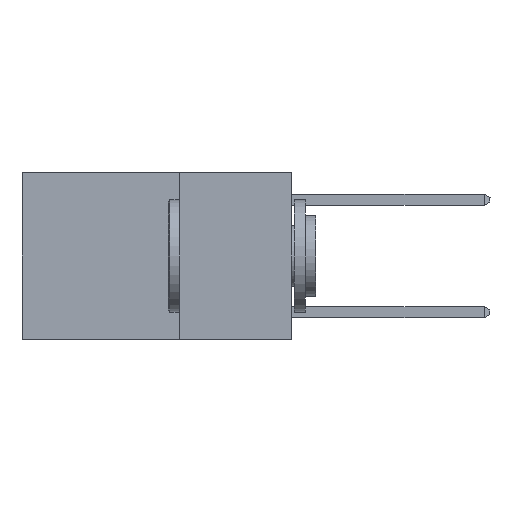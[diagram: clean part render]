
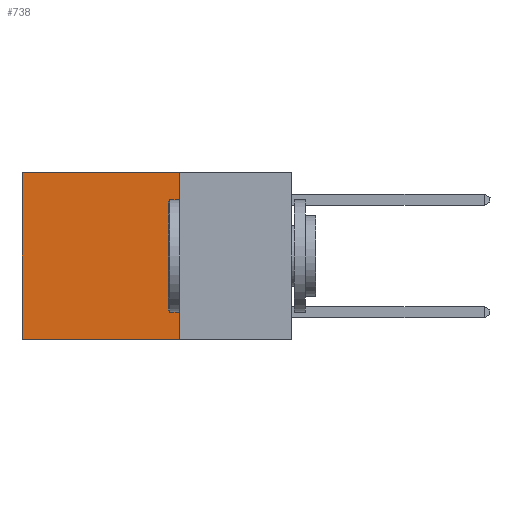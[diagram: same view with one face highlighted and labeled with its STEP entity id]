
A CAD part, left-side view. The second image highlights one B-rep face of the part: STEP entity #738.
In plain terms, the highlighted planar face has unit normal (-1, 0, 0).
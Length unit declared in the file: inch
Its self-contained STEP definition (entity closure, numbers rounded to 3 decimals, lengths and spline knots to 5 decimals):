
#738 = ADVANCED_FACE ( 'NONE', ( #3414 ), #1247, .F. ) ;
#775 = CARTESIAN_POINT ( 'NONE',  ( 0.2625, 0.25, -0.37 ) ) ;
#836 = DIRECTION ( 'NONE',  ( 0., 0., -1. ) ) ;
#953 = CARTESIAN_POINT ( 'NONE',  ( 0.2625, 0.25, 0. ) ) ;
#1247 = PLANE ( 'NONE',  #3187 ) ;
#1680 = LINE ( 'NONE', #4099, #3820 ) ;
#2173 = VECTOR ( 'NONE', #8874, 39.37008 ) ;
#2248 = VERTEX_POINT ( 'NONE', #4805 ) ;
#2487 = CARTESIAN_POINT ( 'NONE',  ( 0.2625, 0.25, 0. ) ) ;
#3187 = AXIS2_PLACEMENT_3D ( 'NONE', #953, #3764, #6591 ) ;
#3414 = FACE_OUTER_BOUND ( 'NONE', #8885, .T. ) ;
#3764 = DIRECTION ( 'NONE',  ( 1., 0., 0. ) ) ;
#3820 = VECTOR ( 'NONE', #9763, 39.37008 ) ;
#4099 = CARTESIAN_POINT ( 'NONE',  ( 0.2625, 0.25, 0. ) ) ;
#4259 = VERTEX_POINT ( 'NONE', #7551 ) ;
#4291 = LINE ( 'NONE', #775, #2173 ) ;
#4509 = VECTOR ( 'NONE', #836, 39.37008 ) ;
#4682 = EDGE_CURVE ( 'NONE', #4259, #4924, #7171, .T. ) ;
#4805 = CARTESIAN_POINT ( 'NONE',  ( 0.2625, 0.25, 0. ) ) ;
#4821 = CARTESIAN_POINT ( 'NONE',  ( 0.2625, 0.6, 0. ) ) ;
#4907 = ORIENTED_EDGE ( 'NONE', *, *, #9030, .F. ) ;
#4924 = VERTEX_POINT ( 'NONE', #10030 ) ;
#5450 = ORIENTED_EDGE ( 'NONE', *, *, #8501, .T. ) ;
#6589 = ORIENTED_EDGE ( 'NONE', *, *, #4682, .T. ) ;
#6591 = DIRECTION ( 'NONE',  ( 0., 0., -1. ) ) ;
#7171 = LINE ( 'NONE', #4821, #4509 ) ;
#7551 = CARTESIAN_POINT ( 'NONE',  ( 0.2625, 0.6, 0. ) ) ;
#7829 = LINE ( 'NONE', #2487, #9715 ) ;
#8501 = EDGE_CURVE ( 'NONE', #2248, #4259, #1680, .T. ) ;
#8874 = DIRECTION ( 'NONE',  ( 0., 1., 0. ) ) ;
#8885 = EDGE_LOOP ( 'NONE', ( #6589, #4907, #9508, #5450 ) ) ;
#8936 = DIRECTION ( 'NONE',  ( 0., 0., -1. ) ) ;
#9030 = EDGE_CURVE ( 'NONE', #10457, #4924, #4291, .T. ) ;
#9508 = ORIENTED_EDGE ( 'NONE', *, *, #10047, .F. ) ;
#9715 = VECTOR ( 'NONE', #8936, 39.37008 ) ;
#9763 = DIRECTION ( 'NONE',  ( 0., 1., 0. ) ) ;
#10030 = CARTESIAN_POINT ( 'NONE',  ( 0.2625, 0.6, -0.37 ) ) ;
#10047 = EDGE_CURVE ( 'NONE', #2248, #10457, #7829, .T. ) ;
#10231 = CARTESIAN_POINT ( 'NONE',  ( 0.2625, 0.25, -0.37 ) ) ;
#10457 = VERTEX_POINT ( 'NONE', #10231 ) ;
